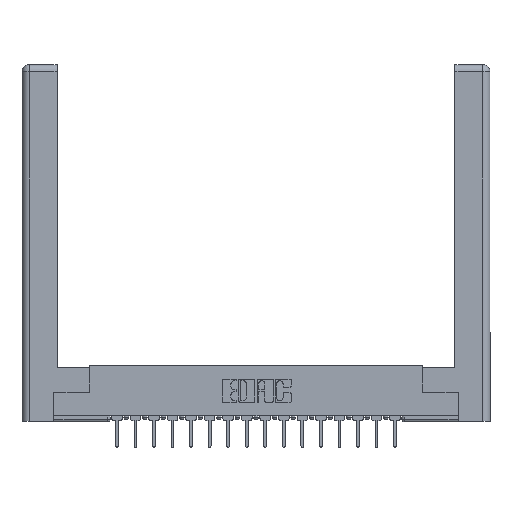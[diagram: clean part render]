
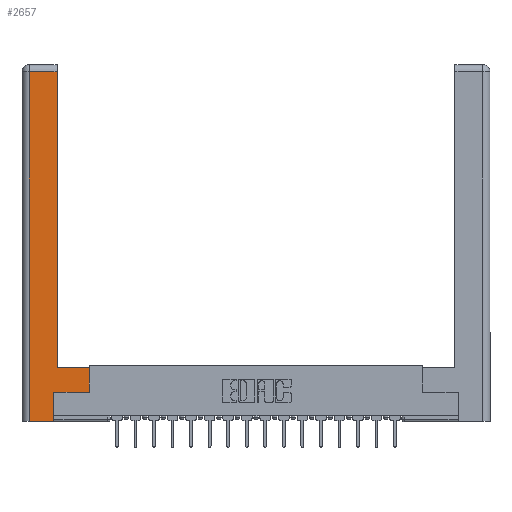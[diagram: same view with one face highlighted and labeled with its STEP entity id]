
A CAD part, top view. The second image highlights one B-rep face of the part: STEP entity #2657.
In plain terms, the highlighted planar face has unit normal (0, 0, 1).
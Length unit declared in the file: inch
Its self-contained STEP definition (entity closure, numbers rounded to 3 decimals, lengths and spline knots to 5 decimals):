
#49 = ORIENTED_EDGE ( 'NONE', *, *, #1973, .T. ) ;
#956 = VECTOR ( 'NONE', #2196, 39.37008 ) ;
#1966 = VERTEX_POINT ( 'NONE', #5716 ) ;
#1973 = EDGE_CURVE ( 'NONE', #7426, #15450, #7919, .T. ) ;
#2196 = DIRECTION ( 'NONE',  ( 0., 1., 0. ) ) ;
#2291 = LINE ( 'NONE', #18110, #956 ) ;
#2367 = DIRECTION ( 'NONE',  ( 0., 0., -1. ) ) ;
#2657 = ADVANCED_FACE ( 'NONE', ( #11629 ), #3907, .F. ) ;
#2867 = ORIENTED_EDGE ( 'NONE', *, *, #3274, .T. ) ;
#3212 = EDGE_CURVE ( 'NONE', #13214, #6997, #4136, .T. ) ;
#3242 = LINE ( 'NONE', #10782, #4512 ) ;
#3274 = EDGE_CURVE ( 'NONE', #4714, #13214, #2291, .T. ) ;
#3342 = ORIENTED_EDGE ( 'NONE', *, *, #3212, .T. ) ;
#3618 = VERTEX_POINT ( 'NONE', #7974 ) ;
#3907 = PLANE ( 'NONE',  #18802 ) ;
#4136 = LINE ( 'NONE', #8596, #18108 ) ;
#4500 = VECTOR ( 'NONE', #6071, 39.37008 ) ;
#4512 = VECTOR ( 'NONE', #15313, 39.37008 ) ;
#4714 = VERTEX_POINT ( 'NONE', #18412 ) ;
#4819 = ORIENTED_EDGE ( 'NONE', *, *, #13023, .T. ) ;
#5716 = CARTESIAN_POINT ( 'NONE',  ( 0.265, 0.245, 0. ) ) ;
#5975 = EDGE_LOOP ( 'NONE', ( #8189, #49, #4819, #9443, #19276, #16149, #2867, #3342 ) ) ;
#6071 = DIRECTION ( 'NONE',  ( 1., 0., 0. ) ) ;
#6131 = CARTESIAN_POINT ( 'NONE',  ( 0.295, 0.45, 0. ) ) ;
#6521 = LINE ( 'NONE', #8139, #16387 ) ;
#6654 = CARTESIAN_POINT ( 'NONE',  ( 0.0615, 2.94, 0. ) ) ;
#6997 = VERTEX_POINT ( 'NONE', #6131 ) ;
#7133 = CARTESIAN_POINT ( 'NONE',  ( 0.295, 2.94, 0. ) ) ;
#7426 = VERTEX_POINT ( 'NONE', #7133 ) ;
#7919 = LINE ( 'NONE', #15427, #17891 ) ;
#7974 = CARTESIAN_POINT ( 'NONE',  ( 0.265, 0., 0. ) ) ;
#8020 = LINE ( 'NONE', #12781, #18218 ) ;
#8084 = VECTOR ( 'NONE', #8499, 39.37008 ) ;
#8139 = CARTESIAN_POINT ( 'NONE',  ( 0.565, 0.245, 0. ) ) ;
#8189 = ORIENTED_EDGE ( 'NONE', *, *, #16265, .T. ) ;
#8499 = DIRECTION ( 'NONE',  ( 0., 1., 0. ) ) ;
#8571 = DIRECTION ( 'NONE',  ( -1., 0., 0. ) ) ;
#8596 = CARTESIAN_POINT ( 'NONE',  ( 0.295, 0.45, 0. ) ) ;
#9094 = EDGE_CURVE ( 'NONE', #1966, #4714, #6521, .T. ) ;
#9204 = LINE ( 'NONE', #12244, #4500 ) ;
#9443 = ORIENTED_EDGE ( 'NONE', *, *, #10341, .T. ) ;
#9658 = CARTESIAN_POINT ( 'NONE',  ( 0.565, 0.45, 0. ) ) ;
#10236 = DIRECTION ( 'NONE',  ( -1., 0., 0. ) ) ;
#10341 = EDGE_CURVE ( 'NONE', #13606, #3618, #9204, .T. ) ;
#10782 = CARTESIAN_POINT ( 'NONE',  ( 0.0615, 0., 0. ) ) ;
#11629 = FACE_OUTER_BOUND ( 'NONE', #5975, .T. ) ;
#11752 = LINE ( 'NONE', #11860, #8084 ) ;
#11860 = CARTESIAN_POINT ( 'NONE',  ( 0.265, 0.245, 0. ) ) ;
#11982 = EDGE_CURVE ( 'NONE', #3618, #1966, #11752, .T. ) ;
#12244 = CARTESIAN_POINT ( 'NONE',  ( 0.265, 0., 0. ) ) ;
#12781 = CARTESIAN_POINT ( 'NONE',  ( 0.295, 3., 0. ) ) ;
#13023 = EDGE_CURVE ( 'NONE', #15450, #13606, #3242, .T. ) ;
#13214 = VERTEX_POINT ( 'NONE', #9658 ) ;
#13606 = VERTEX_POINT ( 'NONE', #19114 ) ;
#13917 = DIRECTION ( 'NONE',  ( -1., 0., 0. ) ) ;
#14196 = DIRECTION ( 'NONE',  ( 0., 1., 0. ) ) ;
#15313 = DIRECTION ( 'NONE',  ( 0., -1., 0. ) ) ;
#15427 = CARTESIAN_POINT ( 'NONE',  ( 0.0615, 2.94, 0. ) ) ;
#15450 = VERTEX_POINT ( 'NONE', #6654 ) ;
#16149 = ORIENTED_EDGE ( 'NONE', *, *, #9094, .T. ) ;
#16257 = CARTESIAN_POINT ( 'NONE',  ( 0., 0., 0. ) ) ;
#16265 = EDGE_CURVE ( 'NONE', #6997, #7426, #8020, .T. ) ;
#16387 = VECTOR ( 'NONE', #18566, 39.37008 ) ;
#17891 = VECTOR ( 'NONE', #13917, 39.37008 ) ;
#18108 = VECTOR ( 'NONE', #10236, 39.37008 ) ;
#18110 = CARTESIAN_POINT ( 'NONE',  ( 0.565, 0.45, 0. ) ) ;
#18218 = VECTOR ( 'NONE', #14196, 39.37008 ) ;
#18412 = CARTESIAN_POINT ( 'NONE',  ( 0.565, 0.245, 0. ) ) ;
#18566 = DIRECTION ( 'NONE',  ( 1., 0., 0. ) ) ;
#18802 = AXIS2_PLACEMENT_3D ( 'NONE', #16257, #2367, #8571 ) ;
#19114 = CARTESIAN_POINT ( 'NONE',  ( 0.0615, 0., 0. ) ) ;
#19276 = ORIENTED_EDGE ( 'NONE', *, *, #11982, .T. ) ;
